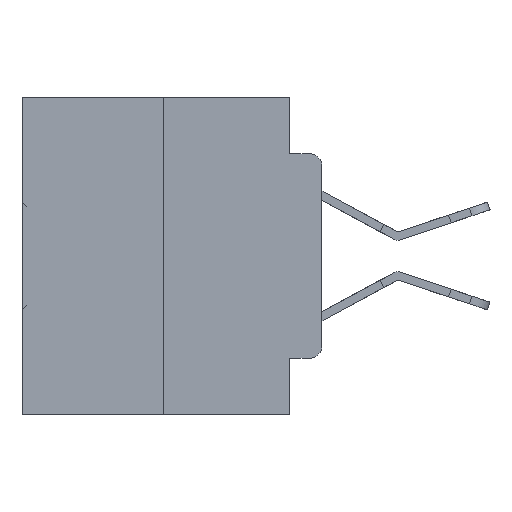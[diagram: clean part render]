
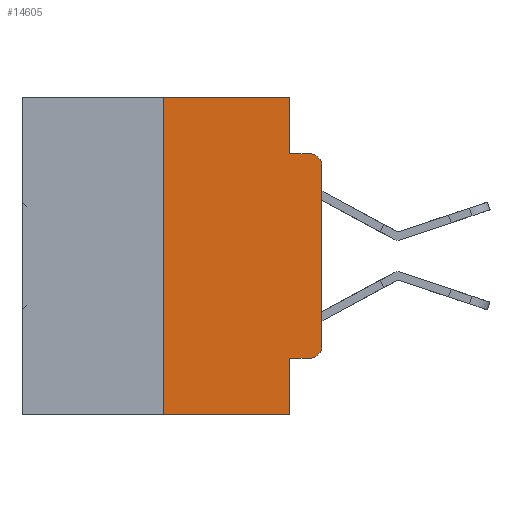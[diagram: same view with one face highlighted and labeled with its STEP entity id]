
A CAD part, left-side view. The second image highlights one B-rep face of the part: STEP entity #14605.
In plain terms, the highlighted planar face has unit normal (-1, 0, 0).
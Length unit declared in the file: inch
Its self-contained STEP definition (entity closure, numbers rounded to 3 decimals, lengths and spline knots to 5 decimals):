
#711 = AXIS2_PLACEMENT_3D ( 'NONE', #32344, #15646, #35147 ) ;
#1175 = VECTOR ( 'NONE', #11643, 39.37008 ) ;
#1828 = DIRECTION ( 'NONE',  ( -1., 0., 0. ) ) ;
#2005 = ORIENTED_EDGE ( 'NONE', *, *, #5204, .T. ) ;
#2012 = EDGE_LOOP ( 'NONE', ( #21706, #22357, #24165, #25211, #20782, #34238, #17835, #17867, #2005, #5800 ) ) ;
#3597 = VECTOR ( 'NONE', #29587, 39.37008 ) ;
#4561 = CARTESIAN_POINT ( 'NONE',  ( 0., 0.25, 0. ) ) ;
#4765 = CARTESIAN_POINT ( 'NONE',  ( 0., 0.051, -0.0885 ) ) ;
#5161 = LINE ( 'NONE', #13858, #34963 ) ;
#5204 = EDGE_CURVE ( 'NONE', #18265, #33291, #11453, .T. ) ;
#5789 = CARTESIAN_POINT ( 'NONE',  ( 0., 0.051, -0.4115 ) ) ;
#5800 = ORIENTED_EDGE ( 'NONE', *, *, #20395, .T. ) ;
#5903 = CARTESIAN_POINT ( 'NONE',  ( 0., 0.473, 0. ) ) ;
#6035 = FACE_OUTER_BOUND ( 'NONE', #2012, .T. ) ;
#6265 = PLANE ( 'NONE',  #29872 ) ;
#6388 = DIRECTION ( 'NONE',  ( 1., 0., 0. ) ) ;
#7829 = VECTOR ( 'NONE', #28839, 39.37008 ) ;
#9444 = DIRECTION ( 'NONE',  ( 0., -1., 0. ) ) ;
#10210 = CARTESIAN_POINT ( 'NONE',  ( 0., 0.051, -0.5 ) ) ;
#10337 = VECTOR ( 'NONE', #18497, 39.37008 ) ;
#10365 = CARTESIAN_POINT ( 'NONE',  ( 0., 0., -0.1085 ) ) ;
#11077 = LINE ( 'NONE', #35143, #3597 ) ;
#11453 = LINE ( 'NONE', #26349, #15054 ) ;
#11643 = DIRECTION ( 'NONE',  ( 0., -1., 0. ) ) ;
#12107 = CARTESIAN_POINT ( 'NONE',  ( 0., 0.25, 0. ) ) ;
#12109 = LINE ( 'NONE', #35135, #10337 ) ;
#13205 = VERTEX_POINT ( 'NONE', #32782 ) ;
#13858 = CARTESIAN_POINT ( 'NONE',  ( 0., 0., 0. ) ) ;
#14541 = EDGE_CURVE ( 'NONE', #22229, #32968, #15327, .T. ) ;
#14605 = ADVANCED_FACE ( 'NONE', ( #6035 ), #6265, .F. ) ;
#15054 = VECTOR ( 'NONE', #9444, 39.37008 ) ;
#15327 = LINE ( 'NONE', #5903, #1175 ) ;
#15342 = LINE ( 'NONE', #23231, #7829 ) ;
#15351 = EDGE_CURVE ( 'NONE', #17386, #18669, #12109, .T. ) ;
#15646 = DIRECTION ( 'NONE',  ( -1., 0., 0. ) ) ;
#16102 = LINE ( 'NONE', #12107, #22687 ) ;
#17171 = EDGE_CURVE ( 'NONE', #28996, #22229, #16102, .T. ) ;
#17386 = VERTEX_POINT ( 'NONE', #4765 ) ;
#17406 = VERTEX_POINT ( 'NONE', #10365 ) ;
#17835 = ORIENTED_EDGE ( 'NONE', *, *, #31696, .T. ) ;
#17867 = ORIENTED_EDGE ( 'NONE', *, *, #20984, .F. ) ;
#18265 = VERTEX_POINT ( 'NONE', #5789 ) ;
#18497 = DIRECTION ( 'NONE',  ( 0., -1., 0. ) ) ;
#18669 = VERTEX_POINT ( 'NONE', #35545 ) ;
#18794 = CARTESIAN_POINT ( 'NONE',  ( 0., 0.02, -0.3915 ) ) ;
#20314 = CARTESIAN_POINT ( 'NONE',  ( 0., 0.473, -0.5 ) ) ;
#20395 = EDGE_CURVE ( 'NONE', #33291, #13205, #25722, .T. ) ;
#20689 = DIRECTION ( 'NONE',  ( 0., 0., 1. ) ) ;
#20782 = ORIENTED_EDGE ( 'NONE', *, *, #14541, .F. ) ;
#20984 = EDGE_CURVE ( 'NONE', #18265, #21701, #11077, .T. ) ;
#21590 = DIRECTION ( 'NONE',  ( 0., 0., -1. ) ) ;
#21668 = VECTOR ( 'NONE', #23112, 39.37008 ) ;
#21701 = VERTEX_POINT ( 'NONE', #10210 ) ;
#21706 = ORIENTED_EDGE ( 'NONE', *, *, #35760, .T. ) ;
#22229 = VERTEX_POINT ( 'NONE', #4561 ) ;
#22357 = ORIENTED_EDGE ( 'NONE', *, *, #22845, .T. ) ;
#22687 = VECTOR ( 'NONE', #20689, 39.37008 ) ;
#22845 = EDGE_CURVE ( 'NONE', #17406, #18669, #31583, .T. ) ;
#23112 = DIRECTION ( 'NONE',  ( 0., -1., 0. ) ) ;
#23231 = CARTESIAN_POINT ( 'NONE',  ( 0., 0.051, 0. ) ) ;
#24165 = ORIENTED_EDGE ( 'NONE', *, *, #15351, .F. ) ;
#24316 = LINE ( 'NONE', #20314, #21668 ) ;
#24654 = EDGE_CURVE ( 'NONE', #32968, #17386, #15342, .T. ) ;
#25094 = DIRECTION ( 'NONE',  ( 0., 0., 1. ) ) ;
#25211 = ORIENTED_EDGE ( 'NONE', *, *, #24654, .F. ) ;
#25722 = CIRCLE ( 'NONE', #30906, 0.02 ) ;
#26098 = DIRECTION ( 'NONE',  ( 0., 0., -1. ) ) ;
#26346 = CARTESIAN_POINT ( 'NONE',  ( 0., 0.051, 0. ) ) ;
#26349 = CARTESIAN_POINT ( 'NONE',  ( 0., 0.051, -0.4115 ) ) ;
#28839 = DIRECTION ( 'NONE',  ( 0., 0., -1. ) ) ;
#28996 = VERTEX_POINT ( 'NONE', #36074 ) ;
#29587 = DIRECTION ( 'NONE',  ( 0., 0., -1. ) ) ;
#29872 = AXIS2_PLACEMENT_3D ( 'NONE', #34326, #6388, #26098 ) ;
#30906 = AXIS2_PLACEMENT_3D ( 'NONE', #18794, #1828, #21590 ) ;
#31583 = CIRCLE ( 'NONE', #711, 0.02 ) ;
#31696 = EDGE_CURVE ( 'NONE', #28996, #21701, #24316, .T. ) ;
#32344 = CARTESIAN_POINT ( 'NONE',  ( 0., 0.02, -0.1085 ) ) ;
#32782 = CARTESIAN_POINT ( 'NONE',  ( 0., 0., -0.3915 ) ) ;
#32968 = VERTEX_POINT ( 'NONE', #26346 ) ;
#33291 = VERTEX_POINT ( 'NONE', #35899 ) ;
#34238 = ORIENTED_EDGE ( 'NONE', *, *, #17171, .F. ) ;
#34326 = CARTESIAN_POINT ( 'NONE',  ( 0., 0.473, 0. ) ) ;
#34963 = VECTOR ( 'NONE', #25094, 39.37008 ) ;
#35135 = CARTESIAN_POINT ( 'NONE',  ( 0., 0.051, -0.0885 ) ) ;
#35143 = CARTESIAN_POINT ( 'NONE',  ( 0., 0.051, 0. ) ) ;
#35147 = DIRECTION ( 'NONE',  ( 0., 0., -1. ) ) ;
#35545 = CARTESIAN_POINT ( 'NONE',  ( 0., 0.02, -0.0885 ) ) ;
#35760 = EDGE_CURVE ( 'NONE', #13205, #17406, #5161, .T. ) ;
#35899 = CARTESIAN_POINT ( 'NONE',  ( 0., 0.02, -0.4115 ) ) ;
#36074 = CARTESIAN_POINT ( 'NONE',  ( 0., 0.25, -0.5 ) ) ;
